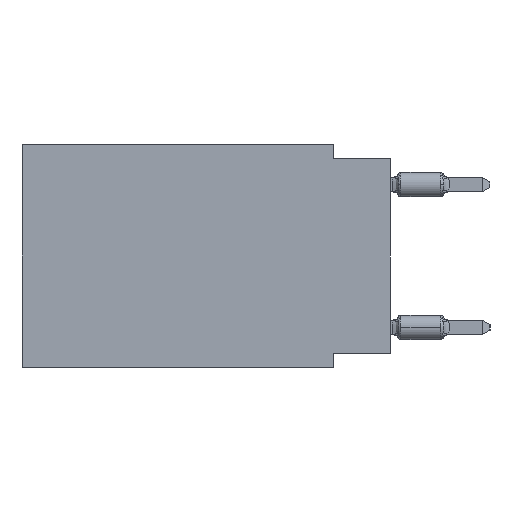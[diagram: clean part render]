
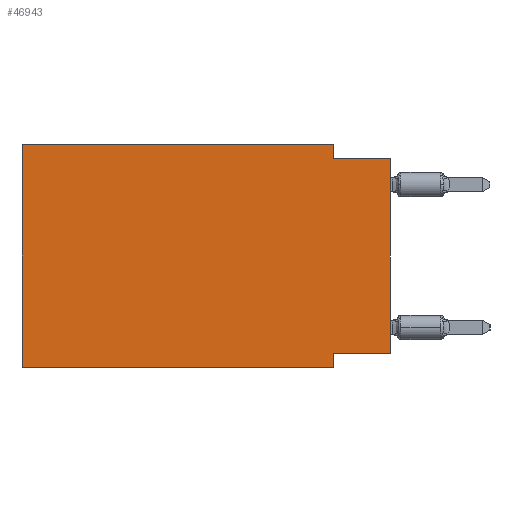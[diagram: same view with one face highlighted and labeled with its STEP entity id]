
A CAD part, left-side view. The second image highlights one B-rep face of the part: STEP entity #46943.
In plain terms, the highlighted planar face has unit normal (-1, 0, 0).
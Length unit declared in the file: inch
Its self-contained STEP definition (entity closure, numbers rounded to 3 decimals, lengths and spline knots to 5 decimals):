
#548 = VECTOR ( 'NONE', #54273, 39.37008 ) ;
#1671 = DIRECTION ( 'NONE',  ( 0., 0., -1. ) ) ;
#2242 = CARTESIAN_POINT ( 'NONE',  ( 0., 0.1, 0. ) ) ;
#2966 = EDGE_CURVE ( 'NONE', #5471, #52884, #26759, .T. ) ;
#3038 = VERTEX_POINT ( 'NONE', #29055 ) ;
#3367 = ORIENTED_EDGE ( 'NONE', *, *, #9539, .F. ) ;
#4770 = EDGE_CURVE ( 'NONE', #5471, #28598, #19372, .T. ) ;
#4804 = ORIENTED_EDGE ( 'NONE', *, *, #25264, .F. ) ;
#5325 = ORIENTED_EDGE ( 'NONE', *, *, #2966, .T. ) ;
#5471 = VERTEX_POINT ( 'NONE', #14773 ) ;
#6931 = EDGE_CURVE ( 'NONE', #33170, #44014, #46768, .T. ) ;
#7254 = DIRECTION ( 'NONE',  ( 0., 1., 0. ) ) ;
#9539 = EDGE_CURVE ( 'NONE', #28598, #48114, #34247, .T. ) ;
#10019 = DIRECTION ( 'NONE',  ( 0., 0., 1. ) ) ;
#10711 = DIRECTION ( 'NONE',  ( 0., 0., 1. ) ) ;
#12089 = ORIENTED_EDGE ( 'NONE', *, *, #49024, .F. ) ;
#13706 = CARTESIAN_POINT ( 'NONE',  ( 0., 0., -0.025 ) ) ;
#14162 = DIRECTION ( 'NONE',  ( 0., 0., -1. ) ) ;
#14660 = CARTESIAN_POINT ( 'NONE',  ( 0., 0.1, -0.39 ) ) ;
#14773 = CARTESIAN_POINT ( 'NONE',  ( 0., 0.645, -0.39 ) ) ;
#17081 = CARTESIAN_POINT ( 'NONE',  ( 0., 0.1, -0.025 ) ) ;
#17485 = LINE ( 'NONE', #47325, #36635 ) ;
#17614 = ORIENTED_EDGE ( 'NONE', *, *, #25508, .T. ) ;
#18929 = CARTESIAN_POINT ( 'NONE',  ( 0., 0.645, 0. ) ) ;
#19372 = LINE ( 'NONE', #41610, #46364 ) ;
#22633 = ORIENTED_EDGE ( 'NONE', *, *, #31326, .F. ) ;
#24167 = CARTESIAN_POINT ( 'NONE',  ( 0., 0., 0. ) ) ;
#25064 = VECTOR ( 'NONE', #29471, 39.37008 ) ;
#25264 = EDGE_CURVE ( 'NONE', #35222, #3038, #17485, .T. ) ;
#25508 = EDGE_CURVE ( 'NONE', #35222, #44014, #37341, .T. ) ;
#26759 = LINE ( 'NONE', #44604, #548 ) ;
#28474 = ORIENTED_EDGE ( 'NONE', *, *, #6931, .F. ) ;
#28598 = VERTEX_POINT ( 'NONE', #18929 ) ;
#29055 = CARTESIAN_POINT ( 'NONE',  ( 0., 0.1, -0.365 ) ) ;
#29471 = DIRECTION ( 'NONE',  ( 0., -1., 0. ) ) ;
#29773 = DIRECTION ( 'NONE',  ( 0., 0., -1. ) ) ;
#31326 = EDGE_CURVE ( 'NONE', #48114, #33170, #42313, .T. ) ;
#31997 = FACE_OUTER_BOUND ( 'NONE', #45936, .T. ) ;
#32283 = CARTESIAN_POINT ( 'NONE',  ( 0., 0.645, 0. ) ) ;
#33018 = CARTESIAN_POINT ( 'NONE',  ( 0., 0., -0.025 ) ) ;
#33170 = VERTEX_POINT ( 'NONE', #17081 ) ;
#34247 = LINE ( 'NONE', #57099, #57374 ) ;
#35222 = VERTEX_POINT ( 'NONE', #45068 ) ;
#36635 = VECTOR ( 'NONE', #7254, 39.37008 ) ;
#37341 = LINE ( 'NONE', #24167, #55323 ) ;
#37536 = PLANE ( 'NONE',  #51211 ) ;
#39290 = ORIENTED_EDGE ( 'NONE', *, *, #4770, .F. ) ;
#40295 = CARTESIAN_POINT ( 'NONE',  ( 0., 0.1, 0. ) ) ;
#41610 = CARTESIAN_POINT ( 'NONE',  ( 0., 0.645, 0. ) ) ;
#41807 = LINE ( 'NONE', #47049, #46218 ) ;
#42313 = LINE ( 'NONE', #2242, #48339 ) ;
#44014 = VERTEX_POINT ( 'NONE', #13706 ) ;
#44604 = CARTESIAN_POINT ( 'NONE',  ( 0., 0.645, -0.39 ) ) ;
#45068 = CARTESIAN_POINT ( 'NONE',  ( 0., 0., -0.365 ) ) ;
#45936 = EDGE_LOOP ( 'NONE', ( #17614, #28474, #22633, #3367, #39290, #5325, #12089, #4804 ) ) ;
#46218 = VECTOR ( 'NONE', #29773, 39.37008 ) ;
#46364 = VECTOR ( 'NONE', #10019, 39.37008 ) ;
#46768 = LINE ( 'NONE', #33018, #25064 ) ;
#46943 = ADVANCED_FACE ( 'NONE', ( #31997 ), #37536, .F. ) ;
#47049 = CARTESIAN_POINT ( 'NONE',  ( 0., 0.1, -0.39 ) ) ;
#47325 = CARTESIAN_POINT ( 'NONE',  ( 0., 0., -0.365 ) ) ;
#48114 = VERTEX_POINT ( 'NONE', #40295 ) ;
#48339 = VECTOR ( 'NONE', #1671, 39.37008 ) ;
#49024 = EDGE_CURVE ( 'NONE', #3038, #52884, #41807, .T. ) ;
#51211 = AXIS2_PLACEMENT_3D ( 'NONE', #32283, #55390, #14162 ) ;
#52689 = DIRECTION ( 'NONE',  ( 0., -1., 0. ) ) ;
#52884 = VERTEX_POINT ( 'NONE', #14660 ) ;
#54273 = DIRECTION ( 'NONE',  ( 0., -1., 0. ) ) ;
#55323 = VECTOR ( 'NONE', #10711, 39.37008 ) ;
#55390 = DIRECTION ( 'NONE',  ( 1., 0., 0. ) ) ;
#57099 = CARTESIAN_POINT ( 'NONE',  ( 0., 0.645, 0. ) ) ;
#57374 = VECTOR ( 'NONE', #52689, 39.37008 ) ;
